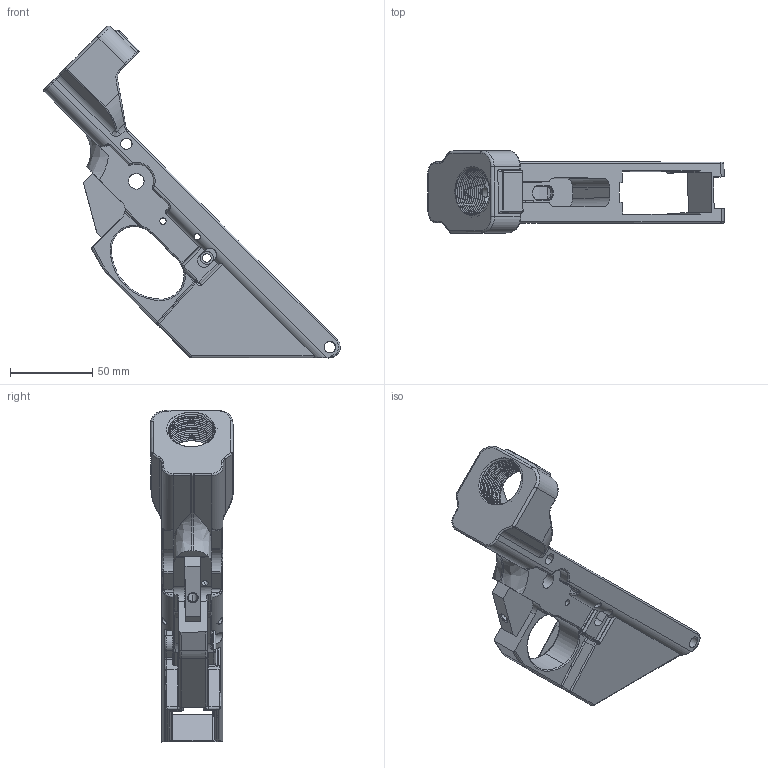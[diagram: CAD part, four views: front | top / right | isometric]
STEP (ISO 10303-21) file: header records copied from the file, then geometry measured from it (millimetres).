
FILE_DESCRIPTION (( 'STEP AP214' ), '1' );
FILE_NAME ('Abraxas_JT_AR-10_V1.STEP', '2015-05-22T11:07:49', ( 'WarFairy' ), ( '' ), 'SwSTEP 2.0', 'SolidWorks 2015', '' );
FILE_SCHEMA (( 'AUTOMOTIVE_DESIGN' ));
Length unit declared in the file: inch
Products named in the file (1): Abraxas_JT_AR-10_V1
Bounding box: 180.12 x 50.23 x 201.59 mm (x, y, z)
Volume: 191944.6 mm3; surface area: 65969.6 mm2
Topology: 1 solids, 1 shells, 475 faces, 1299 edges, 801 vertices
Faces by surface type: cylinder 218, plane 110, bspline 88, torus 49, sphere 6, cone 4
Entity records: 34644 total; most frequent: CARTESIAN_POINT 20264, ORIENTED_EDGE 2560, DIRECTION 2078, EDGE_CURVE 1280, VERTEX_POINT 801, AXIS2_PLACEMENT_3D 777, VECTOR 524, LINE 524
